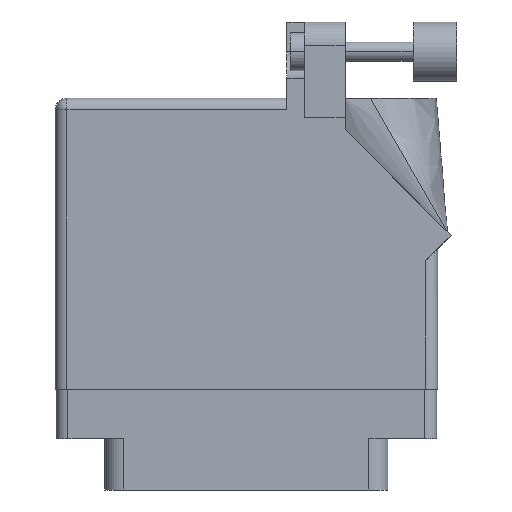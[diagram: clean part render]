
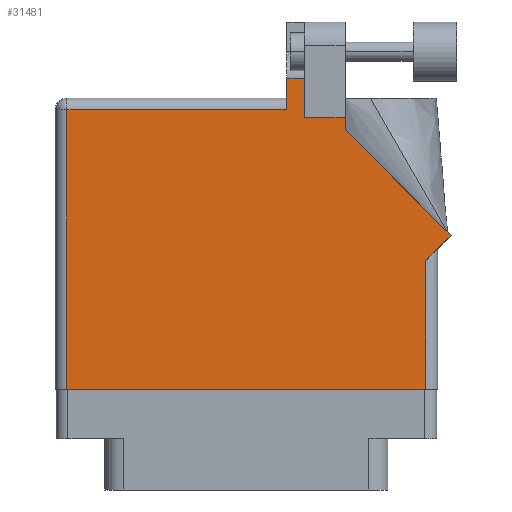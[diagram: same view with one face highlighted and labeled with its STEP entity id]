
A CAD part, front view. The second image highlights one B-rep face of the part: STEP entity #31481.
In plain terms, the highlighted face is planar.
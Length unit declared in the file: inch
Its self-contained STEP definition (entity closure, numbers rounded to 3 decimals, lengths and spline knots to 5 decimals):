
#252 = LINE ( 'NONE', #16736, #32601 ) ;
#696 = LINE ( 'NONE', #6815, #23040 ) ;
#2035 = CARTESIAN_POINT ( 'NONE',  ( 0., 1.53, 0. ) ) ;
#2401 = LINE ( 'NONE', #14391, #23795 ) ;
#2406 = LINE ( 'NONE', #36533, #30016 ) ;
#2727 = DIRECTION ( 'NONE',  ( 0., 1., 0. ) ) ;
#2900 = LINE ( 'NONE', #7648, #23348 ) ;
#2972 = EDGE_CURVE ( 'NONE', #3492, #32062, #252, .T. ) ;
#3332 = DIRECTION ( 'NONE',  ( 0.707, 0.707, 0. ) ) ;
#3492 = VERTEX_POINT ( 'NONE', #27646 ) ;
#3658 = VECTOR ( 'NONE', #2727, 39.37008 ) ;
#4297 = EDGE_CURVE ( 'NONE', #19364, #8055, #25362, .T. ) ;
#4918 = DIRECTION ( 'NONE',  ( 1., 0., 0. ) ) ;
#5235 = VERTEX_POINT ( 'NONE', #7364 ) ;
#5925 = EDGE_CURVE ( 'NONE', #5235, #36313, #11784, .T. ) ;
#6114 = ORIENTED_EDGE ( 'NONE', *, *, #34738, .T. ) ;
#6245 = CARTESIAN_POINT ( 'NONE',  ( 2.01, 0.737, 0. ) ) ;
#6792 = CARTESIAN_POINT ( 'NONE',  ( 1.217, 1.468, 0. ) ) ;
#6815 = CARTESIAN_POINT ( 'NONE',  ( 2.08071, 0.80771, 0. ) ) ;
#6922 = ORIENTED_EDGE ( 'NONE', *, *, #37859, .T. ) ;
#6925 = ORIENTED_EDGE ( 'NONE', *, *, #25749, .T. ) ;
#6936 = CARTESIAN_POINT ( 'NONE',  ( 1.311, 1.6315, 0. ) ) ;
#7364 = CARTESIAN_POINT ( 'NONE',  ( 1.311, 1.43, 0. ) ) ;
#7621 = DIRECTION ( 'NONE',  ( 0., 1., 0. ) ) ;
#7648 = CARTESIAN_POINT ( 'NONE',  ( 1.64177, 1.6315, 0. ) ) ;
#8055 = VERTEX_POINT ( 'NONE', #37073 ) ;
#9939 = EDGE_CURVE ( 'NONE', #14199, #10613, #30959, .T. ) ;
#10355 = EDGE_CURVE ( 'NONE', #8055, #3492, #2401, .T. ) ;
#10501 = CARTESIAN_POINT ( 'NONE',  ( 1.524, 1.36442, 0. ) ) ;
#10613 = VERTEX_POINT ( 'NONE', #24698 ) ;
#10674 = DIRECTION ( 'NONE',  ( -1., 0., 0. ) ) ;
#11405 = LINE ( 'NONE', #14042, #26174 ) ;
#11670 = CARTESIAN_POINT ( 'NONE',  ( 0.062, 0., 0. ) ) ;
#11784 = LINE ( 'NONE', #21187, #3658 ) ;
#13499 = CARTESIAN_POINT ( 'NONE',  ( 0., 1.468, 0. ) ) ;
#13642 = CARTESIAN_POINT ( 'NONE',  ( 0.062, 1.468, 0. ) ) ;
#13883 = VECTOR ( 'NONE', #34209, 39.37008 ) ;
#14042 = CARTESIAN_POINT ( 'NONE',  ( 1.524, 1.43, 0. ) ) ;
#14105 = VECTOR ( 'NONE', #3332, 39.37008 ) ;
#14164 = DIRECTION ( 'NONE',  ( -1., 0., 0. ) ) ;
#14199 = VERTEX_POINT ( 'NONE', #10501 ) ;
#14391 = CARTESIAN_POINT ( 'NONE',  ( 0., 0., 0. ) ) ;
#15258 = ORIENTED_EDGE ( 'NONE', *, *, #38918, .T. ) ;
#16143 = EDGE_CURVE ( 'NONE', #16360, #19274, #2406, .T. ) ;
#16360 = VERTEX_POINT ( 'NONE', #25669 ) ;
#16736 = CARTESIAN_POINT ( 'NONE',  ( 1.948, 0.737, 0. ) ) ;
#17541 = DIRECTION ( 'NONE',  ( 0., -1., 0. ) ) ;
#18106 = VECTOR ( 'NONE', #10674, 39.37008 ) ;
#19046 = AXIS2_PLACEMENT_3D ( 'NONE', #2035, #23309, #35497 ) ;
#19270 = ORIENTED_EDGE ( 'NONE', *, *, #2972, .T. ) ;
#19274 = VERTEX_POINT ( 'NONE', #6792 ) ;
#19364 = VERTEX_POINT ( 'NONE', #13642 ) ;
#19815 = ORIENTED_EDGE ( 'NONE', *, *, #25459, .T. ) ;
#21187 = CARTESIAN_POINT ( 'NONE',  ( 1.311, 1.43, 0. ) ) ;
#23040 = VECTOR ( 'NONE', #37136, 39.37008 ) ;
#23108 = LINE ( 'NONE', #6245, #14105 ) ;
#23309 = DIRECTION ( 'NONE',  ( 0., 0., -1. ) ) ;
#23348 = VECTOR ( 'NONE', #31630, 39.37008 ) ;
#23543 = CARTESIAN_POINT ( 'NONE',  ( 1.948, 0.675, 0. ) ) ;
#23795 = VECTOR ( 'NONE', #4918, 39.37008 ) ;
#24468 = DIRECTION ( 'NONE',  ( 0., -1., 0. ) ) ;
#24698 = CARTESIAN_POINT ( 'NONE',  ( 1.524, 1.43, 0. ) ) ;
#25064 = CARTESIAN_POINT ( 'NONE',  ( 1.524, 1.36442, 0. ) ) ;
#25362 = LINE ( 'NONE', #11670, #27776 ) ;
#25459 = EDGE_CURVE ( 'NONE', #36313, #16360, #2900, .T. ) ;
#25669 = CARTESIAN_POINT ( 'NONE',  ( 1.217, 1.6315, 0. ) ) ;
#25749 = EDGE_CURVE ( 'NONE', #19274, #19364, #27652, .T. ) ;
#25757 = ORIENTED_EDGE ( 'NONE', *, *, #16143, .T. ) ;
#26174 = VECTOR ( 'NONE', #14164, 39.37008 ) ;
#26565 = VERTEX_POINT ( 'NONE', #36383 ) ;
#27646 = CARTESIAN_POINT ( 'NONE',  ( 1.948, 0., 0. ) ) ;
#27652 = LINE ( 'NONE', #13499, #18106 ) ;
#27776 = VECTOR ( 'NONE', #17541, 39.37008 ) ;
#30016 = VECTOR ( 'NONE', #24468, 39.37008 ) ;
#30063 = ORIENTED_EDGE ( 'NONE', *, *, #10355, .T. ) ;
#30093 = ORIENTED_EDGE ( 'NONE', *, *, #4297, .T. ) ;
#30959 = LINE ( 'NONE', #25064, #13883 ) ;
#31481 = ADVANCED_FACE ( 'NONE', ( #38207 ), #35637, .F. ) ;
#31630 = DIRECTION ( 'NONE',  ( -1., 0., 0. ) ) ;
#32062 = VERTEX_POINT ( 'NONE', #23543 ) ;
#32601 = VECTOR ( 'NONE', #7621, 39.37008 ) ;
#34209 = DIRECTION ( 'NONE',  ( 0., 1., 0. ) ) ;
#34738 = EDGE_CURVE ( 'NONE', #10613, #5235, #11405, .T. ) ;
#35497 = DIRECTION ( 'NONE',  ( -1., 0., 0. ) ) ;
#35637 = PLANE ( 'NONE',  #19046 ) ;
#35676 = EDGE_LOOP ( 'NONE', ( #37922, #19815, #25757, #6925, #30093, #30063, #19270, #6922, #15258, #36324, #6114 ) ) ;
#36313 = VERTEX_POINT ( 'NONE', #6936 ) ;
#36324 = ORIENTED_EDGE ( 'NONE', *, *, #9939, .T. ) ;
#36383 = CARTESIAN_POINT ( 'NONE',  ( 2.08071, 0.80771, 0. ) ) ;
#36533 = CARTESIAN_POINT ( 'NONE',  ( 1.217, 1.53, 0. ) ) ;
#37073 = CARTESIAN_POINT ( 'NONE',  ( 0.062, 0., 0. ) ) ;
#37136 = DIRECTION ( 'NONE',  ( -0.707, 0.707, 0. ) ) ;
#37859 = EDGE_CURVE ( 'NONE', #32062, #26565, #23108, .T. ) ;
#37922 = ORIENTED_EDGE ( 'NONE', *, *, #5925, .T. ) ;
#38207 = FACE_OUTER_BOUND ( 'NONE', #35676, .T. ) ;
#38918 = EDGE_CURVE ( 'NONE', #26565, #14199, #696, .T. ) ;
